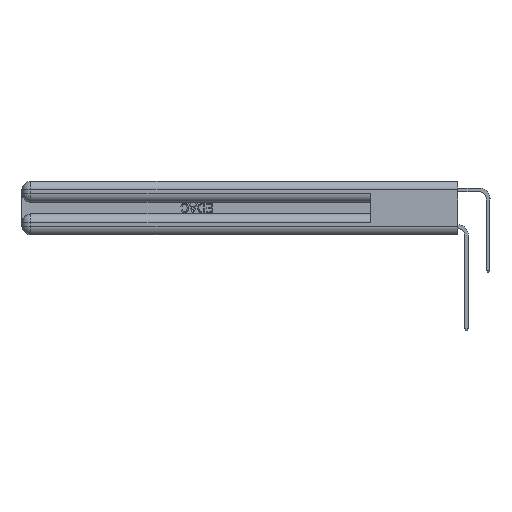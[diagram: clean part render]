
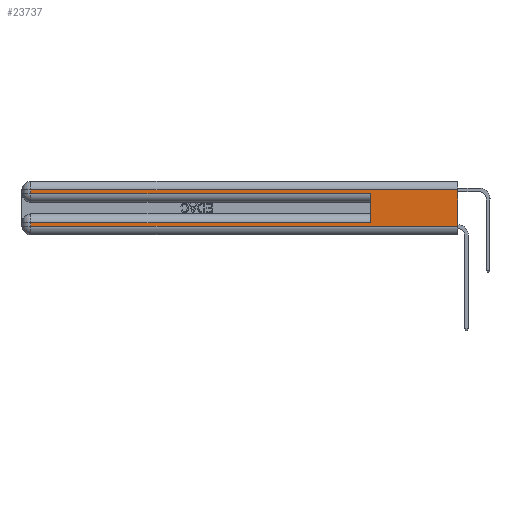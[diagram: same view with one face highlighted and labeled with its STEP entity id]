
A CAD part, left-side view. The second image highlights one B-rep face of the part: STEP entity #23737.
In plain terms, the highlighted planar face has unit normal (-1, 0, 0).
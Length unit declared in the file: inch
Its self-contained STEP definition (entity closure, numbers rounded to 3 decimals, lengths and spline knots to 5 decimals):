
#5 = ORIENTED_EDGE ( 'NONE', *, *, #6799, .T. ) ;
#978 = EDGE_CURVE ( 'NONE', #16795, #4564, #11469, .T. ) ;
#1202 = VECTOR ( 'NONE', #14690, 39.37008 ) ;
#1529 = CARTESIAN_POINT ( 'NONE',  ( 0., 2.94, 0.085 ) ) ;
#1859 = VECTOR ( 'NONE', #33819, 39.37008 ) ;
#2410 = ORIENTED_EDGE ( 'NONE', *, *, #978, .T. ) ;
#2770 = EDGE_LOOP ( 'NONE', ( #5347, #3773, #31755, #34820, #33385, #2410, #35895, #5 ) ) ;
#3674 = VECTOR ( 'NONE', #12684, 39.37008 ) ;
#3773 = ORIENTED_EDGE ( 'NONE', *, *, #16177, .T. ) ;
#4149 = EDGE_CURVE ( 'NONE', #9392, #34896, #8574, .T. ) ;
#4564 = VERTEX_POINT ( 'NONE', #1529 ) ;
#5347 = ORIENTED_EDGE ( 'NONE', *, *, #34921, .F. ) ;
#6708 = CARTESIAN_POINT ( 'NONE',  ( 0., 2.94, 0.37 ) ) ;
#6799 = EDGE_CURVE ( 'NONE', #11330, #15603, #36261, .T. ) ;
#7110 = CARTESIAN_POINT ( 'NONE',  ( 0., 0., 0.37 ) ) ;
#7951 = VECTOR ( 'NONE', #16442, 39.37008 ) ;
#8169 = VECTOR ( 'NONE', #24586, 39.37008 ) ;
#8574 = LINE ( 'NONE', #30093, #8169 ) ;
#9392 = VERTEX_POINT ( 'NONE', #26267 ) ;
#9622 = DIRECTION ( 'NONE',  ( 0., 0., -1. ) ) ;
#9736 = CARTESIAN_POINT ( 'NONE',  ( 0., 0., 0.06 ) ) ;
#10785 = CARTESIAN_POINT ( 'NONE',  ( 0., 0., 0.085 ) ) ;
#11229 = EDGE_CURVE ( 'NONE', #4564, #11330, #14858, .T. ) ;
#11330 = VERTEX_POINT ( 'NONE', #36405 ) ;
#11469 = LINE ( 'NONE', #10785, #7951 ) ;
#12684 = DIRECTION ( 'NONE',  ( 0., 0., 1. ) ) ;
#12907 = CARTESIAN_POINT ( 'NONE',  ( 0., 0.6, 0.085 ) ) ;
#13274 = FACE_OUTER_BOUND ( 'NONE', #2770, .T. ) ;
#13557 = DIRECTION ( 'NONE',  ( 0., 0., -1. ) ) ;
#14256 = AXIS2_PLACEMENT_3D ( 'NONE', #7110, #21092, #9622 ) ;
#14690 = DIRECTION ( 'NONE',  ( 0., 0., -1. ) ) ;
#14858 = LINE ( 'NONE', #6708, #36031 ) ;
#15090 = LINE ( 'NONE', #26832, #3674 ) ;
#15603 = VERTEX_POINT ( 'NONE', #9736 ) ;
#16177 = EDGE_CURVE ( 'NONE', #35212, #35131, #21921, .T. ) ;
#16442 = DIRECTION ( 'NONE',  ( 0., 1., 0. ) ) ;
#16795 = VERTEX_POINT ( 'NONE', #12907 ) ;
#17722 = VECTOR ( 'NONE', #13557, 39.37008 ) ;
#18258 = EDGE_CURVE ( 'NONE', #16795, #34896, #15090, .T. ) ;
#19761 = LINE ( 'NONE', #31818, #1202 ) ;
#21092 = DIRECTION ( 'NONE',  ( 1., 0., 0. ) ) ;
#21612 = CARTESIAN_POINT ( 'NONE',  ( 0., 2.94, 0.31 ) ) ;
#21921 = LINE ( 'NONE', #35186, #29768 ) ;
#22614 = CARTESIAN_POINT ( 'NONE',  ( 0., 0., 0.06 ) ) ;
#23737 = ADVANCED_FACE ( 'NONE', ( #13274 ), #34891, .F. ) ;
#24067 = CARTESIAN_POINT ( 'NONE',  ( 0., 0., 0.31 ) ) ;
#24548 = CARTESIAN_POINT ( 'NONE',  ( 0., 2.94, 0.37 ) ) ;
#24586 = DIRECTION ( 'NONE',  ( 0., -1., 0. ) ) ;
#26267 = CARTESIAN_POINT ( 'NONE',  ( 0., 2.94, 0.285 ) ) ;
#26832 = CARTESIAN_POINT ( 'NONE',  ( 0., 0.6, 0.145 ) ) ;
#28966 = CARTESIAN_POINT ( 'NONE',  ( 0., 0.6, 0.285 ) ) ;
#29242 = DIRECTION ( 'NONE',  ( 0., 0., -1. ) ) ;
#29768 = VECTOR ( 'NONE', #32460, 39.37008 ) ;
#30093 = CARTESIAN_POINT ( 'NONE',  ( 0., 0., 0.285 ) ) ;
#30457 = EDGE_CURVE ( 'NONE', #35131, #9392, #36221, .T. ) ;
#31755 = ORIENTED_EDGE ( 'NONE', *, *, #30457, .T. ) ;
#31818 = CARTESIAN_POINT ( 'NONE',  ( 0., 0., 0.37 ) ) ;
#32460 = DIRECTION ( 'NONE',  ( 0., 1., 0. ) ) ;
#33385 = ORIENTED_EDGE ( 'NONE', *, *, #18258, .F. ) ;
#33819 = DIRECTION ( 'NONE',  ( 0., -1., 0. ) ) ;
#34820 = ORIENTED_EDGE ( 'NONE', *, *, #4149, .T. ) ;
#34891 = PLANE ( 'NONE',  #14256 ) ;
#34896 = VERTEX_POINT ( 'NONE', #28966 ) ;
#34921 = EDGE_CURVE ( 'NONE', #35212, #15603, #19761, .T. ) ;
#35131 = VERTEX_POINT ( 'NONE', #21612 ) ;
#35186 = CARTESIAN_POINT ( 'NONE',  ( 0., 0., 0.31 ) ) ;
#35212 = VERTEX_POINT ( 'NONE', #24067 ) ;
#35895 = ORIENTED_EDGE ( 'NONE', *, *, #11229, .T. ) ;
#36031 = VECTOR ( 'NONE', #29242, 39.37008 ) ;
#36221 = LINE ( 'NONE', #24548, #17722 ) ;
#36261 = LINE ( 'NONE', #22614, #1859 ) ;
#36405 = CARTESIAN_POINT ( 'NONE',  ( 0., 2.94, 0.06 ) ) ;
